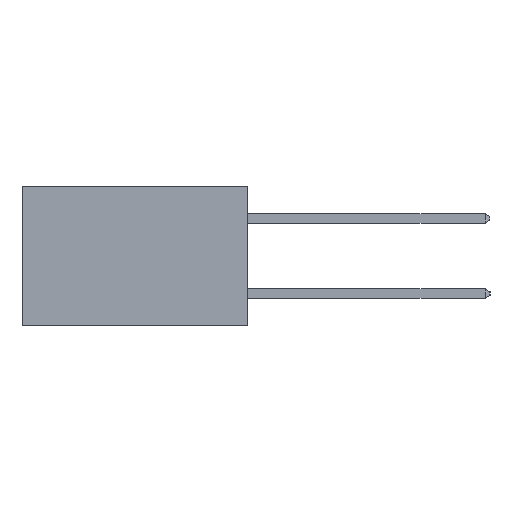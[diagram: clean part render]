
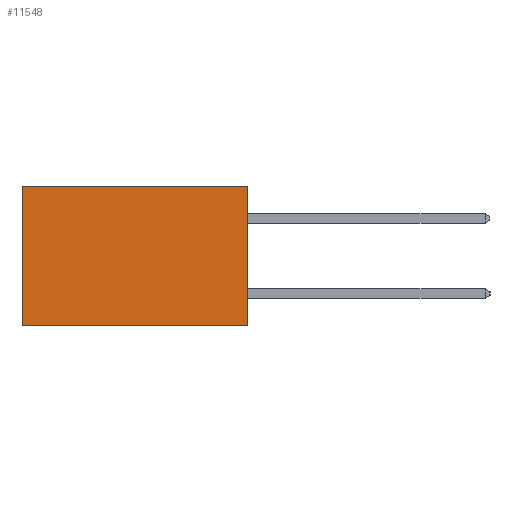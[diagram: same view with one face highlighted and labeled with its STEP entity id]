
A CAD part, left-side view. The second image highlights one B-rep face of the part: STEP entity #11548.
In plain terms, the highlighted planar face has unit normal (-1, 0, 0).
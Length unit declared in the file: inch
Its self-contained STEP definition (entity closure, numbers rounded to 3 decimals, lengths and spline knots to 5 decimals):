
#924 = PLANE ( 'NONE',  #2990 ) ;
#1791 = LINE ( 'NONE', #8520, #14589 ) ;
#1849 = EDGE_CURVE ( 'NONE', #15519, #14958, #6594, .T. ) ;
#2190 = DIRECTION ( 'NONE',  ( 0., 0., -1. ) ) ;
#2990 = AXIS2_PLACEMENT_3D ( 'NONE', #14546, #9653, #2190 ) ;
#3279 = VECTOR ( 'NONE', #4610, 39.37008 ) ;
#3591 = ORIENTED_EDGE ( 'NONE', *, *, #7802, .T. ) ;
#4610 = DIRECTION ( 'NONE',  ( 0., 0., -1. ) ) ;
#4871 = EDGE_CURVE ( 'NONE', #7587, #14958, #14279, .T. ) ;
#4995 = EDGE_LOOP ( 'NONE', ( #13322, #10837, #9213, #3591 ) ) ;
#6197 = DIRECTION ( 'NONE',  ( 0., 1., 0. ) ) ;
#6233 = CARTESIAN_POINT ( 'NONE',  ( 0.2615, 0., 0. ) ) ;
#6594 = LINE ( 'NONE', #8732, #3279 ) ;
#6674 = CARTESIAN_POINT ( 'NONE',  ( 0.2615, 0., 0. ) ) ;
#7348 = CARTESIAN_POINT ( 'NONE',  ( 0.2615, 0.6, -0.37 ) ) ;
#7430 = EDGE_CURVE ( 'NONE', #9888, #7587, #1791, .T. ) ;
#7587 = VERTEX_POINT ( 'NONE', #7605 ) ;
#7605 = CARTESIAN_POINT ( 'NONE',  ( 0.2615, 0., -0.37 ) ) ;
#7802 = EDGE_CURVE ( 'NONE', #9888, #15519, #12910, .T. ) ;
#8520 = CARTESIAN_POINT ( 'NONE',  ( 0.2615, 0., -0.37 ) ) ;
#8570 = DIRECTION ( 'NONE',  ( 0., 0., -1. ) ) ;
#8682 = CARTESIAN_POINT ( 'NONE',  ( 0.2615, 0.6, 0. ) ) ;
#8732 = CARTESIAN_POINT ( 'NONE',  ( 0.2615, 0.6, -0.37 ) ) ;
#9213 = ORIENTED_EDGE ( 'NONE', *, *, #7430, .F. ) ;
#9653 = DIRECTION ( 'NONE',  ( 1., 0., 0. ) ) ;
#9888 = VERTEX_POINT ( 'NONE', #6674 ) ;
#10680 = FACE_OUTER_BOUND ( 'NONE', #4995, .T. ) ;
#10837 = ORIENTED_EDGE ( 'NONE', *, *, #4871, .F. ) ;
#11032 = VECTOR ( 'NONE', #12365, 39.37008 ) ;
#11548 = ADVANCED_FACE ( 'NONE', ( #10680 ), #924, .F. ) ;
#12365 = DIRECTION ( 'NONE',  ( 0., 1., 0. ) ) ;
#12403 = CARTESIAN_POINT ( 'NONE',  ( 0.2615, 0., -0.37 ) ) ;
#12521 = VECTOR ( 'NONE', #6197, 39.37008 ) ;
#12910 = LINE ( 'NONE', #6233, #12521 ) ;
#13322 = ORIENTED_EDGE ( 'NONE', *, *, #1849, .T. ) ;
#14279 = LINE ( 'NONE', #12403, #11032 ) ;
#14546 = CARTESIAN_POINT ( 'NONE',  ( 0.2615, 0., -0.37 ) ) ;
#14589 = VECTOR ( 'NONE', #8570, 39.37008 ) ;
#14958 = VERTEX_POINT ( 'NONE', #7348 ) ;
#15519 = VERTEX_POINT ( 'NONE', #8682 ) ;
